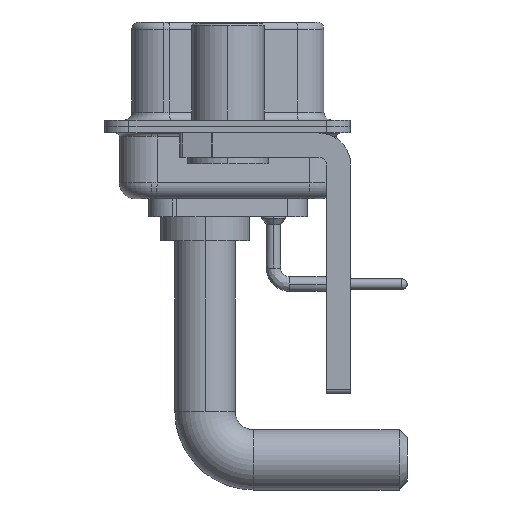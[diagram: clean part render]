
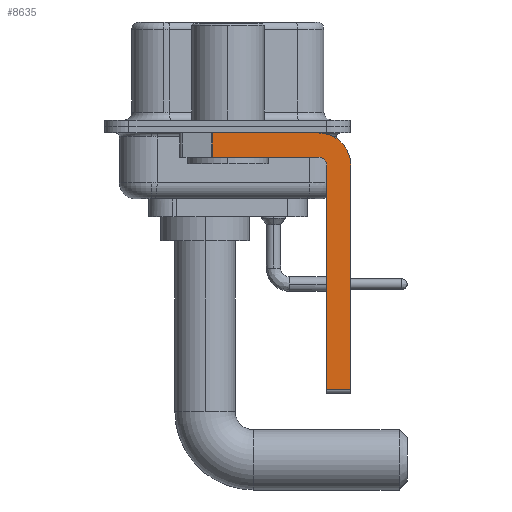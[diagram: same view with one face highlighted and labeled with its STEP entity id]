
A CAD part, left-side view. The second image highlights one B-rep face of the part: STEP entity #8635.
In plain terms, the highlighted planar face has unit normal (-1, 0, 0).
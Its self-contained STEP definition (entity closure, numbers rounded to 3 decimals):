
#169 = VERTEX_POINT ( 'NONE', #13350 ) ;
#756 = VERTEX_POINT ( 'NONE', #6278 ) ;
#882 = CARTESIAN_POINT ( 'NONE',  ( -2.9, 3., -0.4 ) ) ;
#1640 = EDGE_CURVE ( 'NONE', #169, #23171, #22559, .T. ) ;
#1852 = CARTESIAN_POINT ( 'NONE',  ( -2.9, -5.65, -2.4 ) ) ;
#2884 = VERTEX_POINT ( 'NONE', #24673 ) ;
#3677 = CARTESIAN_POINT ( 'NONE',  ( -2.9, -5.65, -2.4 ) ) ;
#4194 = EDGE_LOOP ( 'NONE', ( #24687, #22448, #11910, #19418, #5480, #23747, #17497, #10805 ) ) ;
#4404 = EDGE_CURVE ( 'NONE', #23171, #5558, #5442, .T. ) ;
#5029 = VECTOR ( 'NONE', #25299, 1000. ) ;
#5442 = LINE ( 'NONE', #25459, #22042 ) ;
#5480 = ORIENTED_EDGE ( 'NONE', *, *, #20702, .F. ) ;
#5489 = EDGE_CURVE ( 'NONE', #2884, #19358, #22517, .T. ) ;
#5558 = VERTEX_POINT ( 'NONE', #25157 ) ;
#5933 = LINE ( 'NONE', #15974, #17489 ) ;
#6278 = CARTESIAN_POINT ( 'NONE',  ( -2.9, -6.15, -2.4 ) ) ;
#6671 = LINE ( 'NONE', #14700, #15237 ) ;
#6787 = VERTEX_POINT ( 'NONE', #26252 ) ;
#7293 = CARTESIAN_POINT ( 'NONE',  ( -2.9, 0.978, -1.9 ) ) ;
#7831 = EDGE_CURVE ( 'NONE', #11997, #5558, #6671, .T. ) ;
#8088 = DIRECTION ( 'NONE',  ( 0., 0., -1. ) ) ;
#8635 = ADVANCED_FACE ( 'NONE', ( #15885 ), #24520, .F. ) ;
#9135 = CARTESIAN_POINT ( 'NONE',  ( -2.9, -5.65, -2.4 ) ) ;
#9264 = DIRECTION ( 'NONE',  ( 1., 0., 0. ) ) ;
#10750 = CARTESIAN_POINT ( 'NONE',  ( -2.9, -6.15, -16.35 ) ) ;
#10754 = DIRECTION ( 'NONE',  ( 0., 0., -1. ) ) ;
#10805 = ORIENTED_EDGE ( 'NONE', *, *, #1640, .F. ) ;
#11595 = DIRECTION ( 'NONE',  ( 0., 0., -1. ) ) ;
#11857 = DIRECTION ( 'NONE',  ( 0., 0., 1. ) ) ;
#11910 = ORIENTED_EDGE ( 'NONE', *, *, #25455, .F. ) ;
#11997 = VERTEX_POINT ( 'NONE', #10750 ) ;
#12263 = AXIS2_PLACEMENT_3D ( 'NONE', #1852, #18031, #24265 ) ;
#13350 = CARTESIAN_POINT ( 'NONE',  ( -2.9, -5.65, -0.4 ) ) ;
#13949 = VECTOR ( 'NONE', #11857, 1000. ) ;
#14700 = CARTESIAN_POINT ( 'NONE',  ( -2.9, -5.65, -16.35 ) ) ;
#14738 = CIRCLE ( 'NONE', #22834, 0.5 ) ;
#15237 = VECTOR ( 'NONE', #20979, 1000. ) ;
#15885 = FACE_OUTER_BOUND ( 'NONE', #4194, .T. ) ;
#15974 = CARTESIAN_POINT ( 'NONE',  ( -2.9, -5.65, -1.9 ) ) ;
#15984 = DIRECTION ( 'NONE',  ( -1., 0., 0. ) ) ;
#16002 = LINE ( 'NONE', #23727, #13949 ) ;
#16546 = AXIS2_PLACEMENT_3D ( 'NONE', #9135, #9264, #10754 ) ;
#17489 = VECTOR ( 'NONE', #20122, 1000. ) ;
#17497 = ORIENTED_EDGE ( 'NONE', *, *, #4404, .F. ) ;
#17898 = EDGE_CURVE ( 'NONE', #756, #6787, #14738, .T. ) ;
#18031 = DIRECTION ( 'NONE',  ( 1., 0., 0. ) ) ;
#19041 = VECTOR ( 'NONE', #8088, 1000. ) ;
#19188 = LINE ( 'NONE', #882, #5029 ) ;
#19358 = VERTEX_POINT ( 'NONE', #7293 ) ;
#19418 = ORIENTED_EDGE ( 'NONE', *, *, #17898, .F. ) ;
#20122 = DIRECTION ( 'NONE',  ( 0., 1., 0. ) ) ;
#20251 = DIRECTION ( 'NONE',  ( 0., 0., 1. ) ) ;
#20702 = EDGE_CURVE ( 'NONE', #11997, #756, #16002, .T. ) ;
#20979 = DIRECTION ( 'NONE',  ( 0., -1., 0. ) ) ;
#22042 = VECTOR ( 'NONE', #11595, 1000. ) ;
#22448 = ORIENTED_EDGE ( 'NONE', *, *, #5489, .T. ) ;
#22517 = LINE ( 'NONE', #26381, #19041 ) ;
#22559 = CIRCLE ( 'NONE', #16546, 2. ) ;
#22596 = EDGE_CURVE ( 'NONE', #2884, #169, #19188, .T. ) ;
#22834 = AXIS2_PLACEMENT_3D ( 'NONE', #3677, #15984, #20251 ) ;
#23171 = VERTEX_POINT ( 'NONE', #25527 ) ;
#23727 = CARTESIAN_POINT ( 'NONE',  ( -2.9, -6.15, -16.6 ) ) ;
#23747 = ORIENTED_EDGE ( 'NONE', *, *, #7831, .T. ) ;
#24265 = DIRECTION ( 'NONE',  ( 0., 0., -1. ) ) ;
#24520 = PLANE ( 'NONE',  #12263 ) ;
#24673 = CARTESIAN_POINT ( 'NONE',  ( -2.9, 0.978, -0.4 ) ) ;
#24687 = ORIENTED_EDGE ( 'NONE', *, *, #22596, .F. ) ;
#25157 = CARTESIAN_POINT ( 'NONE',  ( -2.9, -7.65, -16.35 ) ) ;
#25299 = DIRECTION ( 'NONE',  ( 0., -1., 0. ) ) ;
#25455 = EDGE_CURVE ( 'NONE', #6787, #19358, #5933, .T. ) ;
#25459 = CARTESIAN_POINT ( 'NONE',  ( -2.9, -7.65, -2.4 ) ) ;
#25527 = CARTESIAN_POINT ( 'NONE',  ( -2.9, -7.65, -2.4 ) ) ;
#26252 = CARTESIAN_POINT ( 'NONE',  ( -2.9, -5.65, -1.9 ) ) ;
#26381 = CARTESIAN_POINT ( 'NONE',  ( -2.9, 0.978, -1.9 ) ) ;
